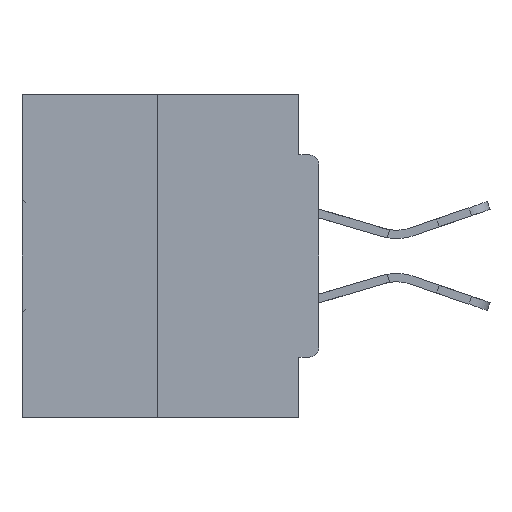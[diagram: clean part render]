
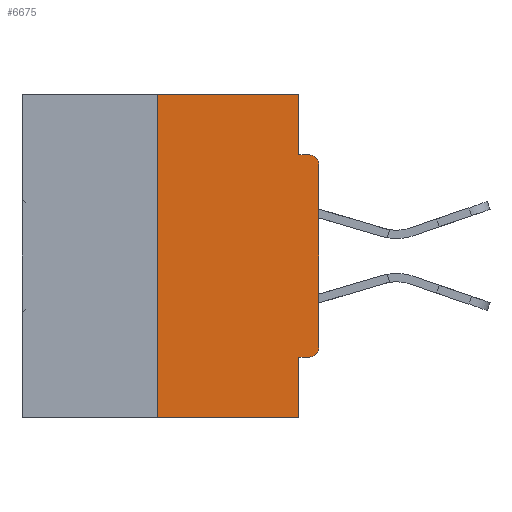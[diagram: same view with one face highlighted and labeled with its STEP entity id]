
A CAD part, left-side view. The second image highlights one B-rep face of the part: STEP entity #6675.
In plain terms, the highlighted planar face has unit normal (-1, 0, 0).
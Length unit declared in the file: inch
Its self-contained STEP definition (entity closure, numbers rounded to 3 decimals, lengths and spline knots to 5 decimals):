
#533 = EDGE_CURVE ( 'NONE', #21049, #6864, #11075, .T. ) ;
#885 = EDGE_CURVE ( 'NONE', #41813, #14109, #21246, .T. ) ;
#1408 = LINE ( 'NONE', #1670, #21282 ) ;
#1670 = CARTESIAN_POINT ( 'NONE',  ( 0., 0., -0.0935 ) ) ;
#1889 = CARTESIAN_POINT ( 'NONE',  ( 0., 0., -0.4065 ) ) ;
#2398 = EDGE_CURVE ( 'NONE', #5992, #24570, #41375, .T. ) ;
#2606 = VERTEX_POINT ( 'NONE', #10698 ) ;
#3939 = EDGE_LOOP ( 'NONE', ( #35879, #41747, #24412, #13131, #20425, #4237, #26608, #39781, #21796, #40189 ) ) ;
#3964 = DIRECTION ( 'NONE',  ( 0., 0., -1. ) ) ;
#4237 = ORIENTED_EDGE ( 'NONE', *, *, #13396, .T. ) ;
#4410 = CIRCLE ( 'NONE', #17667, 0.015 ) ;
#4560 = CARTESIAN_POINT ( 'NONE',  ( 0., 0.031, 0. ) ) ;
#5316 = VECTOR ( 'NONE', #27918, 39.37008 ) ;
#5593 = LINE ( 'NONE', #39276, #22278 ) ;
#5992 = VERTEX_POINT ( 'NONE', #20941 ) ;
#6028 = EDGE_CURVE ( 'NONE', #40323, #21049, #6209, .T. ) ;
#6101 = VECTOR ( 'NONE', #11573, 39.37008 ) ;
#6209 = LINE ( 'NONE', #33884, #40577 ) ;
#6534 = CARTESIAN_POINT ( 'NONE',  ( 0., 0.031, -0.4065 ) ) ;
#6675 = ADVANCED_FACE ( 'NONE', ( #19211 ), #39956, .F. ) ;
#6864 = VERTEX_POINT ( 'NONE', #11022 ) ;
#9568 = CARTESIAN_POINT ( 'NONE',  ( 0., 0.25, 0. ) ) ;
#10698 = CARTESIAN_POINT ( 'NONE',  ( 0., 0.015, -0.0935 ) ) ;
#10879 = EDGE_CURVE ( 'NONE', #6864, #2606, #1408, .T. ) ;
#11022 = CARTESIAN_POINT ( 'NONE',  ( 0., 0.031, -0.0935 ) ) ;
#11075 = LINE ( 'NONE', #24558, #5316 ) ;
#11132 = AXIS2_PLACEMENT_3D ( 'NONE', #30520, #40094, #3964 ) ;
#11573 = DIRECTION ( 'NONE',  ( 0., 1., 0. ) ) ;
#13131 = ORIENTED_EDGE ( 'NONE', *, *, #40426, .F. ) ;
#13376 = CARTESIAN_POINT ( 'NONE',  ( 0., 0.031, -0.5 ) ) ;
#13396 = EDGE_CURVE ( 'NONE', #41813, #5992, #4410, .T. ) ;
#14109 = VERTEX_POINT ( 'NONE', #6534 ) ;
#14180 = DIRECTION ( 'NONE',  ( -1., 0., 0. ) ) ;
#14259 = EDGE_CURVE ( 'NONE', #24570, #2606, #22127, .T. ) ;
#14883 = LINE ( 'NONE', #13376, #40376 ) ;
#15201 = VERTEX_POINT ( 'NONE', #32187 ) ;
#17667 = AXIS2_PLACEMENT_3D ( 'NONE', #29750, #19458, #39494 ) ;
#19211 = FACE_OUTER_BOUND ( 'NONE', #3939, .T. ) ;
#19458 = DIRECTION ( 'NONE',  ( -1., 0., 0. ) ) ;
#20425 = ORIENTED_EDGE ( 'NONE', *, *, #885, .F. ) ;
#20941 = CARTESIAN_POINT ( 'NONE',  ( 0., 0., -0.3915 ) ) ;
#21014 = DIRECTION ( 'NONE',  ( 0., 0., -1. ) ) ;
#21049 = VERTEX_POINT ( 'NONE', #4560 ) ;
#21246 = LINE ( 'NONE', #1889, #6101 ) ;
#21282 = VECTOR ( 'NONE', #30997, 39.37008 ) ;
#21796 = ORIENTED_EDGE ( 'NONE', *, *, #10879, .F. ) ;
#22127 = CIRCLE ( 'NONE', #40548, 0.015 ) ;
#22278 = VECTOR ( 'NONE', #22672, 39.37008 ) ;
#22672 = DIRECTION ( 'NONE',  ( 0., -1., 0. ) ) ;
#23871 = VERTEX_POINT ( 'NONE', #31458 ) ;
#24412 = ORIENTED_EDGE ( 'NONE', *, *, #36468, .T. ) ;
#24558 = CARTESIAN_POINT ( 'NONE',  ( 0., 0.031, 0. ) ) ;
#24570 = VERTEX_POINT ( 'NONE', #29515 ) ;
#26608 = ORIENTED_EDGE ( 'NONE', *, *, #2398, .T. ) ;
#27918 = DIRECTION ( 'NONE',  ( 0., 0., -1. ) ) ;
#28427 = CARTESIAN_POINT ( 'NONE',  ( 0., 0.25, 0. ) ) ;
#29515 = CARTESIAN_POINT ( 'NONE',  ( 0., 0., -0.1085 ) ) ;
#29750 = CARTESIAN_POINT ( 'NONE',  ( 0., 0.015, -0.3915 ) ) ;
#30520 = CARTESIAN_POINT ( 'NONE',  ( 0., 0.46, 0. ) ) ;
#30551 = DIRECTION ( 'NONE',  ( 0., -1., 0. ) ) ;
#30997 = DIRECTION ( 'NONE',  ( 0., -1., 0. ) ) ;
#31458 = CARTESIAN_POINT ( 'NONE',  ( 0., 0.25, -0.5 ) ) ;
#32187 = CARTESIAN_POINT ( 'NONE',  ( 0., 0.031, -0.5 ) ) ;
#33059 = VECTOR ( 'NONE', #34975, 39.37008 ) ;
#33884 = CARTESIAN_POINT ( 'NONE',  ( 0., 0.46, 0. ) ) ;
#34097 = CARTESIAN_POINT ( 'NONE',  ( 0., 0.015, -0.1085 ) ) ;
#34606 = VECTOR ( 'NONE', #36614, 39.37008 ) ;
#34975 = DIRECTION ( 'NONE',  ( 0., 0., 1. ) ) ;
#35879 = ORIENTED_EDGE ( 'NONE', *, *, #6028, .F. ) ;
#36373 = DIRECTION ( 'NONE',  ( 0., 0., -1. ) ) ;
#36468 = EDGE_CURVE ( 'NONE', #23871, #15201, #5593, .T. ) ;
#36614 = DIRECTION ( 'NONE',  ( 0., 0., 1. ) ) ;
#36964 = CARTESIAN_POINT ( 'NONE',  ( 0., 0.015, -0.4065 ) ) ;
#39276 = CARTESIAN_POINT ( 'NONE',  ( 0., 0.46, -0.5 ) ) ;
#39494 = DIRECTION ( 'NONE',  ( 0., 0., -1. ) ) ;
#39781 = ORIENTED_EDGE ( 'NONE', *, *, #14259, .T. ) ;
#39790 = CARTESIAN_POINT ( 'NONE',  ( 0., 0., 0. ) ) ;
#39956 = PLANE ( 'NONE',  #11132 ) ;
#40094 = DIRECTION ( 'NONE',  ( 1., 0., 0. ) ) ;
#40189 = ORIENTED_EDGE ( 'NONE', *, *, #533, .F. ) ;
#40323 = VERTEX_POINT ( 'NONE', #9568 ) ;
#40376 = VECTOR ( 'NONE', #36373, 39.37008 ) ;
#40426 = EDGE_CURVE ( 'NONE', #14109, #15201, #14883, .T. ) ;
#40548 = AXIS2_PLACEMENT_3D ( 'NONE', #34097, #14180, #21014 ) ;
#40577 = VECTOR ( 'NONE', #30551, 39.37008 ) ;
#41375 = LINE ( 'NONE', #39790, #34606 ) ;
#41405 = EDGE_CURVE ( 'NONE', #23871, #40323, #42967, .T. ) ;
#41747 = ORIENTED_EDGE ( 'NONE', *, *, #41405, .F. ) ;
#41813 = VERTEX_POINT ( 'NONE', #36964 ) ;
#42967 = LINE ( 'NONE', #28427, #33059 ) ;
